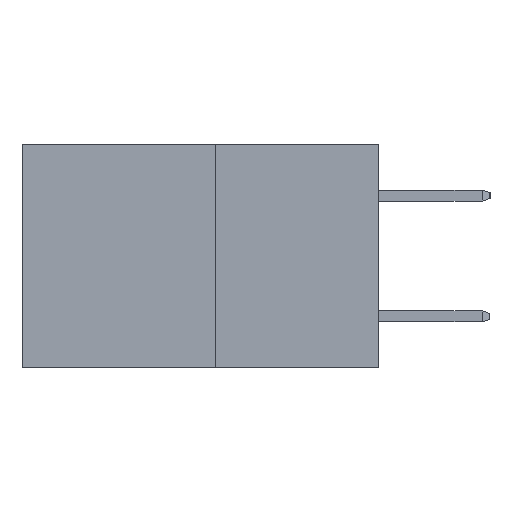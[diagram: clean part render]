
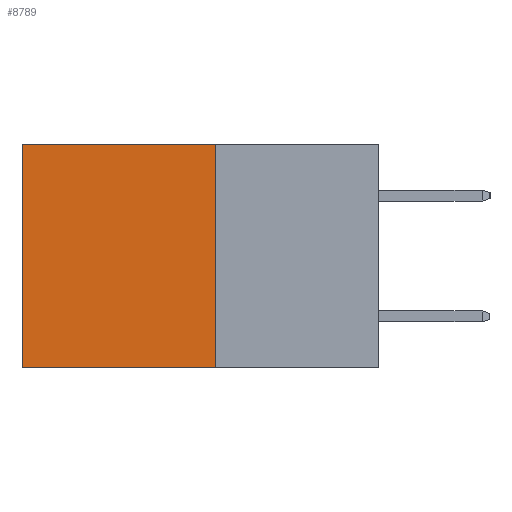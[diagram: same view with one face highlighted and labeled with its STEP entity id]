
A CAD part, left-side view. The second image highlights one B-rep face of the part: STEP entity #8789.
In plain terms, the highlighted planar face has unit normal (-1, 0, 0).
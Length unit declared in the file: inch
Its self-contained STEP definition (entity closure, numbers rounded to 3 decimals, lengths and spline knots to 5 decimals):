
#169 = DIRECTION ( 'NONE',  ( 0., 1., 0. ) ) ;
#359 = LINE ( 'NONE', #8490, #2979 ) ;
#1416 = CARTESIAN_POINT ( 'NONE',  ( 0.277, 0.27, -0.37 ) ) ;
#1803 = DIRECTION ( 'NONE',  ( 0., 0., -1. ) ) ;
#1845 = ORIENTED_EDGE ( 'NONE', *, *, #12961, .T. ) ;
#1932 = VERTEX_POINT ( 'NONE', #6252 ) ;
#2075 = ORIENTED_EDGE ( 'NONE', *, *, #10844, .F. ) ;
#2900 = CARTESIAN_POINT ( 'NONE',  ( 0.277, 0.27, -0.37 ) ) ;
#2979 = VECTOR ( 'NONE', #1803, 39.37008 ) ;
#4055 = AXIS2_PLACEMENT_3D ( 'NONE', #6189, #13800, #7310 ) ;
#4365 = FACE_OUTER_BOUND ( 'NONE', #6163, .T. ) ;
#4495 = VERTEX_POINT ( 'NONE', #8876 ) ;
#5149 = DIRECTION ( 'NONE',  ( 0., 1., 0. ) ) ;
#5267 = CARTESIAN_POINT ( 'NONE',  ( 0.277, 0.27, 0. ) ) ;
#5395 = ORIENTED_EDGE ( 'NONE', *, *, #8858, .F. ) ;
#5853 = VECTOR ( 'NONE', #169, 39.37008 ) ;
#5923 = DIRECTION ( 'NONE',  ( 0., 0., -1. ) ) ;
#6116 = EDGE_CURVE ( 'NONE', #7688, #4495, #11689, .T. ) ;
#6163 = EDGE_LOOP ( 'NONE', ( #1845, #5395, #2075, #6620 ) ) ;
#6189 = CARTESIAN_POINT ( 'NONE',  ( 0.277, 0.27, -0.37 ) ) ;
#6252 = CARTESIAN_POINT ( 'NONE',  ( 0.277, 0.27, -0.37 ) ) ;
#6620 = ORIENTED_EDGE ( 'NONE', *, *, #6116, .T. ) ;
#6648 = LINE ( 'NONE', #2900, #12117 ) ;
#7310 = DIRECTION ( 'NONE',  ( 0., 0., -1. ) ) ;
#7688 = VERTEX_POINT ( 'NONE', #5267 ) ;
#8019 = CARTESIAN_POINT ( 'NONE',  ( 0.277, 0.27, 0. ) ) ;
#8490 = CARTESIAN_POINT ( 'NONE',  ( 0.277, 0.59, -0.37 ) ) ;
#8789 = ADVANCED_FACE ( 'NONE', ( #4365 ), #12741, .F. ) ;
#8858 = EDGE_CURVE ( 'NONE', #1932, #12136, #6648, .T. ) ;
#8876 = CARTESIAN_POINT ( 'NONE',  ( 0.277, 0.59, 0. ) ) ;
#10320 = VECTOR ( 'NONE', #5923, 39.37008 ) ;
#10648 = LINE ( 'NONE', #1416, #10320 ) ;
#10844 = EDGE_CURVE ( 'NONE', #7688, #1932, #10648, .T. ) ;
#11546 = CARTESIAN_POINT ( 'NONE',  ( 0.277, 0.59, -0.37 ) ) ;
#11689 = LINE ( 'NONE', #8019, #5853 ) ;
#12117 = VECTOR ( 'NONE', #5149, 39.37008 ) ;
#12136 = VERTEX_POINT ( 'NONE', #11546 ) ;
#12741 = PLANE ( 'NONE',  #4055 ) ;
#12961 = EDGE_CURVE ( 'NONE', #4495, #12136, #359, .T. ) ;
#13800 = DIRECTION ( 'NONE',  ( 1., 0., 0. ) ) ;
